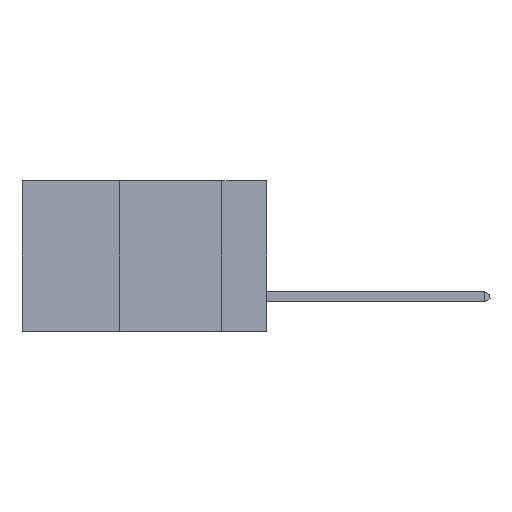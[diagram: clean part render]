
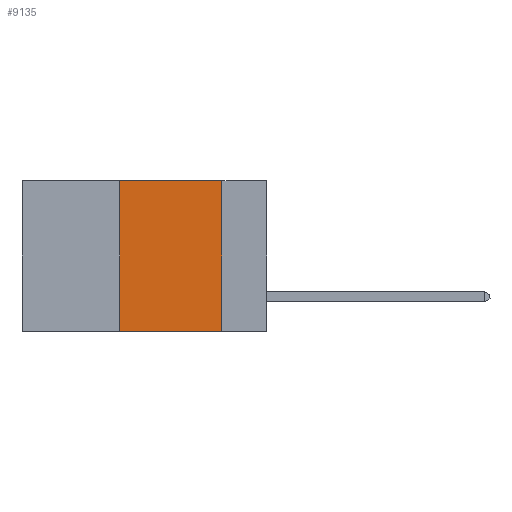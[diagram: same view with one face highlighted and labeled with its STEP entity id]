
A CAD part, left-side view. The second image highlights one B-rep face of the part: STEP entity #9135.
In plain terms, the highlighted planar face has unit normal (-1, 0, 0).
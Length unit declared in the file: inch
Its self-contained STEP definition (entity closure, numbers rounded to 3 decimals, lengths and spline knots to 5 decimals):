
#71 = LINE ( 'NONE', #713, #4569 ) ;
#309 = LINE ( 'NONE', #7566, #13849 ) ;
#713 = CARTESIAN_POINT ( 'NONE',  ( 0., 0.11, 0. ) ) ;
#766 = ORIENTED_EDGE ( 'NONE', *, *, #10206, .T. ) ;
#793 = DIRECTION ( 'NONE',  ( 0., 0., -1. ) ) ;
#1027 = VERTEX_POINT ( 'NONE', #6289 ) ;
#2793 = VERTEX_POINT ( 'NONE', #4707 ) ;
#3733 = DIRECTION ( 'NONE',  ( 0., 0., 1. ) ) ;
#4569 = VECTOR ( 'NONE', #6132, 39.37008 ) ;
#4685 = DIRECTION ( 'NONE',  ( 0., -1., 0. ) ) ;
#4707 = CARTESIAN_POINT ( 'NONE',  ( 0., 0.11, 0. ) ) ;
#4836 = PLANE ( 'NONE',  #13684 ) ;
#5117 = DIRECTION ( 'NONE',  ( 1., 0., 0. ) ) ;
#5132 = LINE ( 'NONE', #8066, #11525 ) ;
#5194 = CARTESIAN_POINT ( 'NONE',  ( 0., 0.36, 0. ) ) ;
#5839 = FACE_OUTER_BOUND ( 'NONE', #6809, .T. ) ;
#6132 = DIRECTION ( 'NONE',  ( 0., 0., -1. ) ) ;
#6289 = CARTESIAN_POINT ( 'NONE',  ( 0., 0.36, -0.37 ) ) ;
#6809 = EDGE_LOOP ( 'NONE', ( #12267, #12697, #9406, #766 ) ) ;
#6881 = VERTEX_POINT ( 'NONE', #5194 ) ;
#7566 = CARTESIAN_POINT ( 'NONE',  ( 0., 0.6, -0.37 ) ) ;
#8066 = CARTESIAN_POINT ( 'NONE',  ( 0., 0.36, 0. ) ) ;
#9135 = ADVANCED_FACE ( 'NONE', ( #5839 ), #4836, .F. ) ;
#9406 = ORIENTED_EDGE ( 'NONE', *, *, #10006, .F. ) ;
#9428 = VERTEX_POINT ( 'NONE', #13847 ) ;
#10006 = EDGE_CURVE ( 'NONE', #1027, #6881, #5132, .T. ) ;
#10206 = EDGE_CURVE ( 'NONE', #1027, #9428, #309, .T. ) ;
#11487 = LINE ( 'NONE', #12020, #11836 ) ;
#11515 = EDGE_CURVE ( 'NONE', #6881, #2793, #11487, .T. ) ;
#11525 = VECTOR ( 'NONE', #3733, 39.37008 ) ;
#11762 = DIRECTION ( 'NONE',  ( 0., -1., 0. ) ) ;
#11836 = VECTOR ( 'NONE', #4685, 39.37008 ) ;
#12020 = CARTESIAN_POINT ( 'NONE',  ( 0., 0.6, 0. ) ) ;
#12267 = ORIENTED_EDGE ( 'NONE', *, *, #13027, .F. ) ;
#12347 = CARTESIAN_POINT ( 'NONE',  ( 0., 0.6, 0. ) ) ;
#12697 = ORIENTED_EDGE ( 'NONE', *, *, #11515, .F. ) ;
#13027 = EDGE_CURVE ( 'NONE', #2793, #9428, #71, .T. ) ;
#13684 = AXIS2_PLACEMENT_3D ( 'NONE', #12347, #5117, #793 ) ;
#13847 = CARTESIAN_POINT ( 'NONE',  ( 0., 0.11, -0.37 ) ) ;
#13849 = VECTOR ( 'NONE', #11762, 39.37008 ) ;
